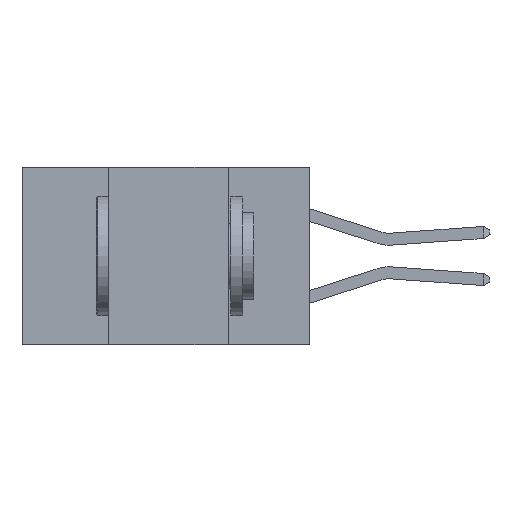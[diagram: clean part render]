
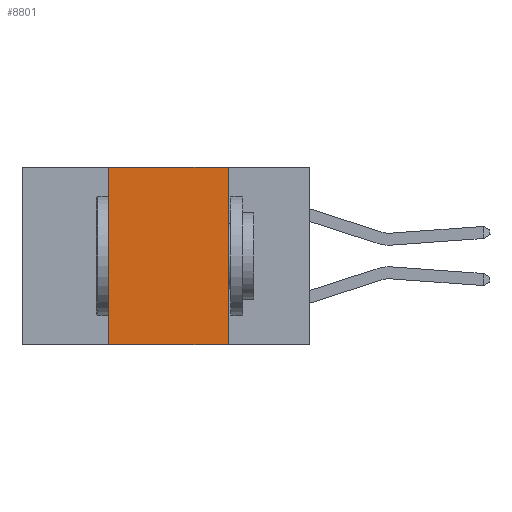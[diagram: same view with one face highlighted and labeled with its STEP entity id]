
A CAD part, left-side view. The second image highlights one B-rep face of the part: STEP entity #8801.
In plain terms, the highlighted planar face has unit normal (-1, 0, 0).
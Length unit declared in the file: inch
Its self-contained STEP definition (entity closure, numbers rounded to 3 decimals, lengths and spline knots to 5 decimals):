
#83 = LINE ( 'NONE', #3350, #11494 ) ;
#215 = DIRECTION ( 'NONE',  ( 0., -1., 0. ) ) ;
#276 = LINE ( 'NONE', #350, #13578 ) ;
#350 = CARTESIAN_POINT ( 'NONE',  ( 0., 0.17, -0.37 ) ) ;
#430 = EDGE_CURVE ( 'NONE', #12150, #10658, #276, .T. ) ;
#991 = VERTEX_POINT ( 'NONE', #13555 ) ;
#2347 = CARTESIAN_POINT ( 'NONE',  ( 0., 0.6, -0.37 ) ) ;
#2607 = EDGE_CURVE ( 'NONE', #991, #12150, #83, .T. ) ;
#2632 = CARTESIAN_POINT ( 'NONE',  ( 0., 0.42, -0.37 ) ) ;
#2843 = DIRECTION ( 'NONE',  ( 0., 0., 1. ) ) ;
#3350 = CARTESIAN_POINT ( 'NONE',  ( 0., 0.6, 0. ) ) ;
#3409 = LINE ( 'NONE', #2347, #6811 ) ;
#3733 = ORIENTED_EDGE ( 'NONE', *, *, #2607, .F. ) ;
#3930 = EDGE_LOOP ( 'NONE', ( #8066, #3733, #13627, #8344 ) ) ;
#4231 = CARTESIAN_POINT ( 'NONE',  ( 0., 0.6, 0. ) ) ;
#6603 = CARTESIAN_POINT ( 'NONE',  ( 0., 0.42, -0.37 ) ) ;
#6811 = VECTOR ( 'NONE', #215, 39.37008 ) ;
#6975 = DIRECTION ( 'NONE',  ( 0., 0., -1. ) ) ;
#7321 = DIRECTION ( 'NONE',  ( 1., 0., 0. ) ) ;
#7394 = FACE_OUTER_BOUND ( 'NONE', #3930, .T. ) ;
#8066 = ORIENTED_EDGE ( 'NONE', *, *, #430, .F. ) ;
#8344 = ORIENTED_EDGE ( 'NONE', *, *, #8484, .T. ) ;
#8452 = DIRECTION ( 'NONE',  ( 0., 0., -1. ) ) ;
#8484 = EDGE_CURVE ( 'NONE', #9416, #10658, #3409, .T. ) ;
#8589 = CARTESIAN_POINT ( 'NONE',  ( 0., 0.17, -0.37 ) ) ;
#8801 = ADVANCED_FACE ( 'NONE', ( #7394 ), #12687, .F. ) ;
#8919 = DIRECTION ( 'NONE',  ( 0., -1., 0. ) ) ;
#9325 = LINE ( 'NONE', #2632, #11604 ) ;
#9416 = VERTEX_POINT ( 'NONE', #6603 ) ;
#9810 = EDGE_CURVE ( 'NONE', #9416, #991, #9325, .T. ) ;
#10636 = CARTESIAN_POINT ( 'NONE',  ( 0., 0.17, 0. ) ) ;
#10658 = VERTEX_POINT ( 'NONE', #8589 ) ;
#11494 = VECTOR ( 'NONE', #8919, 39.37008 ) ;
#11604 = VECTOR ( 'NONE', #2843, 39.37008 ) ;
#12150 = VERTEX_POINT ( 'NONE', #10636 ) ;
#12461 = AXIS2_PLACEMENT_3D ( 'NONE', #4231, #7321, #8452 ) ;
#12687 = PLANE ( 'NONE',  #12461 ) ;
#13555 = CARTESIAN_POINT ( 'NONE',  ( 0., 0.42, 0. ) ) ;
#13578 = VECTOR ( 'NONE', #6975, 39.37008 ) ;
#13627 = ORIENTED_EDGE ( 'NONE', *, *, #9810, .F. ) ;
